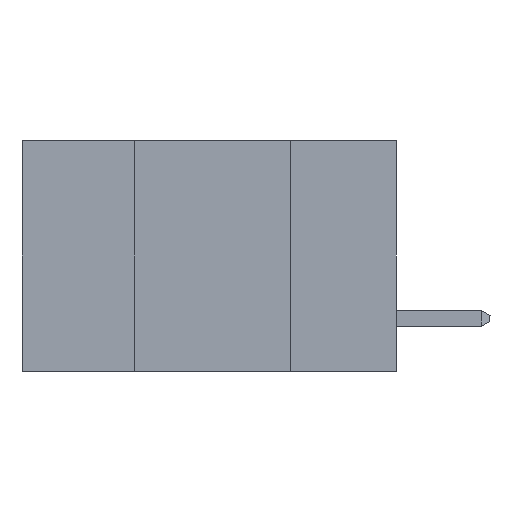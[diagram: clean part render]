
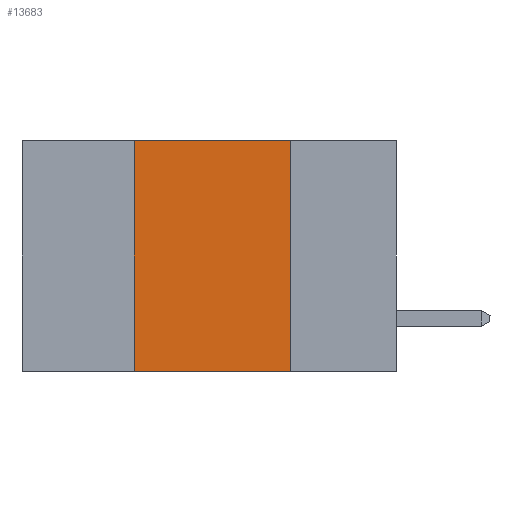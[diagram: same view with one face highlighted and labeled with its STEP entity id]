
A CAD part, left-side view. The second image highlights one B-rep face of the part: STEP entity #13683.
In plain terms, the highlighted planar face has unit normal (-1, 0, 0).
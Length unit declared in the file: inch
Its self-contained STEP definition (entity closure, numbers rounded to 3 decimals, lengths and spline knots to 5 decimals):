
#375 = CARTESIAN_POINT ( 'NONE',  ( 0., 0.42, -0.37 ) ) ;
#512 = ORIENTED_EDGE ( 'NONE', *, *, #15926, .F. ) ;
#1049 = PLANE ( 'NONE',  #7429 ) ;
#1062 = CARTESIAN_POINT ( 'NONE',  ( 0., 0.17, -0.37 ) ) ;
#1573 = CARTESIAN_POINT ( 'NONE',  ( 0., 0.17, -0.37 ) ) ;
#1859 = ORIENTED_EDGE ( 'NONE', *, *, #6137, .T. ) ;
#1904 = DIRECTION ( 'NONE',  ( 0., 0., 1. ) ) ;
#2394 = CARTESIAN_POINT ( 'NONE',  ( 0., 0.17, 0. ) ) ;
#2637 = VERTEX_POINT ( 'NONE', #2394 ) ;
#3010 = LINE ( 'NONE', #1573, #13288 ) ;
#4204 = FACE_OUTER_BOUND ( 'NONE', #15859, .T. ) ;
#4433 = EDGE_CURVE ( 'NONE', #9988, #13009, #14866, .T. ) ;
#4657 = CARTESIAN_POINT ( 'NONE',  ( 0., 0.6, -0.37 ) ) ;
#4997 = ORIENTED_EDGE ( 'NONE', *, *, #4433, .F. ) ;
#5598 = LINE ( 'NONE', #8085, #12061 ) ;
#6137 = EDGE_CURVE ( 'NONE', #9988, #10694, #10563, .T. ) ;
#6880 = CARTESIAN_POINT ( 'NONE',  ( 0., 0.6, 0. ) ) ;
#7429 = AXIS2_PLACEMENT_3D ( 'NONE', #6880, #15825, #18496 ) ;
#8085 = CARTESIAN_POINT ( 'NONE',  ( 0., 0.6, 0. ) ) ;
#9012 = CARTESIAN_POINT ( 'NONE',  ( 0., 0.42, -0.37 ) ) ;
#9988 = VERTEX_POINT ( 'NONE', #9012 ) ;
#10563 = LINE ( 'NONE', #4657, #11244 ) ;
#10612 = CARTESIAN_POINT ( 'NONE',  ( 0., 0.42, 0. ) ) ;
#10694 = VERTEX_POINT ( 'NONE', #1062 ) ;
#11244 = VECTOR ( 'NONE', #14847, 39.37008 ) ;
#12061 = VECTOR ( 'NONE', #18548, 39.37008 ) ;
#12297 = ORIENTED_EDGE ( 'NONE', *, *, #16140, .F. ) ;
#13009 = VERTEX_POINT ( 'NONE', #10612 ) ;
#13189 = DIRECTION ( 'NONE',  ( 0., 0., -1. ) ) ;
#13288 = VECTOR ( 'NONE', #13189, 39.37008 ) ;
#13683 = ADVANCED_FACE ( 'NONE', ( #4204 ), #1049, .F. ) ;
#14847 = DIRECTION ( 'NONE',  ( 0., -1., 0. ) ) ;
#14866 = LINE ( 'NONE', #375, #18664 ) ;
#15825 = DIRECTION ( 'NONE',  ( 1., 0., 0. ) ) ;
#15859 = EDGE_LOOP ( 'NONE', ( #12297, #512, #4997, #1859 ) ) ;
#15926 = EDGE_CURVE ( 'NONE', #13009, #2637, #5598, .T. ) ;
#16140 = EDGE_CURVE ( 'NONE', #2637, #10694, #3010, .T. ) ;
#18496 = DIRECTION ( 'NONE',  ( 0., 0., -1. ) ) ;
#18548 = DIRECTION ( 'NONE',  ( 0., -1., 0. ) ) ;
#18664 = VECTOR ( 'NONE', #1904, 39.37008 ) ;
